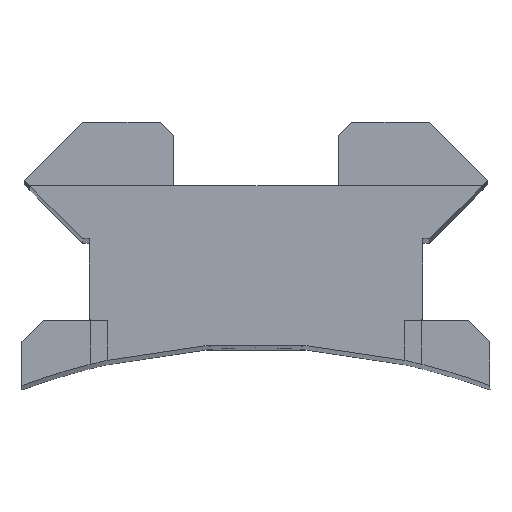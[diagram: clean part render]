
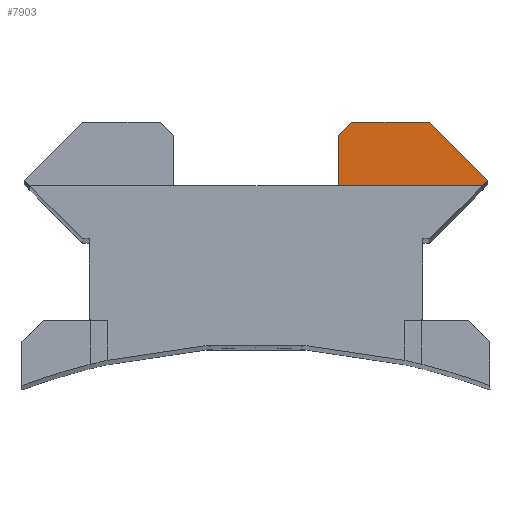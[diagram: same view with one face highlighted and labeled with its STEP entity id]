
A CAD part, top view. The second image highlights one B-rep face of the part: STEP entity #7903.
In plain terms, the highlighted planar face has unit normal (0, 0, 1).
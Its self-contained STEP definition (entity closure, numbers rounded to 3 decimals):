
#1750 = PLANE('',#1751);
#1751 = AXIS2_PLACEMENT_3D('',#1752,#1753,#1754);
#1752 = CARTESIAN_POINT('',(8.153,3.835,0.));
#1753 = DIRECTION('',(0.707,-0.707,0.));
#1754 = DIRECTION('',(0.,0.,-1.));
#2114 = PLANE('',#2115);
#2115 = AXIS2_PLACEMENT_3D('',#2116,#2117,#2118);
#2116 = CARTESIAN_POINT('',(10.897,6.325,-172.669));
#2117 = DIRECTION('',(0.,-1.,0.));
#2118 = DIRECTION('',(0.,0.,-1.));
#4170 = VERTEX_POINT('',#4171);
#4171 = CARTESIAN_POINT('',(10.897,6.579,-31.394));
#4185 = PLANE('',#4186);
#4186 = AXIS2_PLACEMENT_3D('',#4187,#4188,#4189);
#4187 = CARTESIAN_POINT('',(10.897,6.579,0.));
#4188 = DIRECTION('',(0.707,0.707,0.));
#4189 = DIRECTION('',(0.,0.,-1.));
#4197 = EDGE_CURVE('',#4170,#4198,#4200,.T.);
#4198 = VERTEX_POINT('',#4199);
#4199 = CARTESIAN_POINT('',(10.643,6.325,-31.394));
#4200 = SURFACE_CURVE('',#4201,(#4205,#4212),.PCURVE_S1.);
#4201 = LINE('',#4202,#4203);
#4202 = CARTESIAN_POINT('',(10.897,6.579,-31.394));
#4203 = VECTOR('',#4204,1.);
#4204 = DIRECTION('',(-0.707,-0.707,0.));
#4205 = PCURVE('',#1750,#4206);
#4206 = DEFINITIONAL_REPRESENTATION('',(#4207),#4211);
#4207 = LINE('',#4208,#4209);
#4208 = CARTESIAN_POINT('',(31.394,3.879));
#4209 = VECTOR('',#4210,1.);
#4210 = DIRECTION('',(0.,-1.));
#4211 = ( GEOMETRIC_REPRESENTATION_CONTEXT(2) 
PARAMETRIC_REPRESENTATION_CONTEXT() REPRESENTATION_CONTEXT('2D SPACE',''
  ) );
#4212 = PCURVE('',#4213,#4218);
#4213 = PLANE('',#4214);
#4214 = AXIS2_PLACEMENT_3D('',#4215,#4216,#4217);
#4215 = CARTESIAN_POINT('',(10.897,6.325,-31.394));
#4216 = DIRECTION('',(0.,0.,-1.));
#4217 = DIRECTION('',(-1.,0.,0.));
#4218 = DEFINITIONAL_REPRESENTATION('',(#4219),#4223);
#4219 = LINE('',#4220,#4221);
#4220 = CARTESIAN_POINT('',(0.,0.254));
#4221 = VECTOR('',#4222,1.);
#4222 = DIRECTION('',(0.707,-0.707));
#4223 = ( GEOMETRIC_REPRESENTATION_CONTEXT(2) 
PARAMETRIC_REPRESENTATION_CONTEXT() REPRESENTATION_CONTEXT('2D SPACE',''
  ) );
#5285 = VERTEX_POINT('',#5286);
#5286 = CARTESIAN_POINT('',(3.862,6.325,-31.394));
#5300 = PLANE('',#5301);
#5301 = AXIS2_PLACEMENT_3D('',#5302,#5303,#5304);
#5302 = CARTESIAN_POINT('',(3.862,6.325,0.));
#5303 = DIRECTION('',(1.,0.,0.));
#5304 = DIRECTION('',(0.,0.,-1.));
#5312 = EDGE_CURVE('',#4198,#5285,#5313,.T.);
#5313 = SURFACE_CURVE('',#5314,(#5318,#5325),.PCURVE_S1.);
#5314 = LINE('',#5315,#5316);
#5315 = CARTESIAN_POINT('',(10.643,6.325,-31.394));
#5316 = VECTOR('',#5317,1.);
#5317 = DIRECTION('',(-1.,0.,0.));
#5318 = PCURVE('',#2114,#5319);
#5319 = DEFINITIONAL_REPRESENTATION('',(#5320),#5324);
#5320 = LINE('',#5321,#5322);
#5321 = CARTESIAN_POINT('',(-141.275,-0.254));
#5322 = VECTOR('',#5323,1.);
#5323 = DIRECTION('',(0.,-1.));
#5324 = ( GEOMETRIC_REPRESENTATION_CONTEXT(2) 
PARAMETRIC_REPRESENTATION_CONTEXT() REPRESENTATION_CONTEXT('2D SPACE',''
  ) );
#5325 = PCURVE('',#4213,#5326);
#5326 = DEFINITIONAL_REPRESENTATION('',(#5327),#5331);
#5327 = LINE('',#5328,#5329);
#5328 = CARTESIAN_POINT('',(0.254,0.));
#5329 = VECTOR('',#5330,1.);
#5330 = DIRECTION('',(1.,0.));
#5331 = ( GEOMETRIC_REPRESENTATION_CONTEXT(2) 
PARAMETRIC_REPRESENTATION_CONTEXT() REPRESENTATION_CONTEXT('2D SPACE',''
  ) );
#7903 = ADVANCED_FACE('',(#7904),#4213,.F.);
#7904 = FACE_BOUND('',#7905,.T.);
#7905 = EDGE_LOOP('',(#7906,#7936,#7957,#7958,#7959,#7982));
#7906 = ORIENTED_EDGE('',*,*,#7907,.F.);
#7907 = EDGE_CURVE('',#7908,#7910,#7912,.T.);
#7908 = VERTEX_POINT('',#7909);
#7909 = CARTESIAN_POINT('',(3.862,8.687,-31.394));
#7910 = VERTEX_POINT('',#7911);
#7911 = CARTESIAN_POINT('',(4.497,9.322,-31.394));
#7912 = SURFACE_CURVE('',#7913,(#7917,#7924),.PCURVE_S1.);
#7913 = LINE('',#7914,#7915);
#7914 = CARTESIAN_POINT('',(3.862,8.687,-31.394));
#7915 = VECTOR('',#7916,1.);
#7916 = DIRECTION('',(0.707,0.707,0.));
#7917 = PCURVE('',#4213,#7918);
#7918 = DEFINITIONAL_REPRESENTATION('',(#7919),#7923);
#7919 = LINE('',#7920,#7921);
#7920 = CARTESIAN_POINT('',(7.034,2.362));
#7921 = VECTOR('',#7922,1.);
#7922 = DIRECTION('',(-0.707,0.707));
#7923 = ( GEOMETRIC_REPRESENTATION_CONTEXT(2) 
PARAMETRIC_REPRESENTATION_CONTEXT() REPRESENTATION_CONTEXT('2D SPACE',''
  ) );
#7924 = PCURVE('',#7925,#7930);
#7925 = PLANE('',#7926);
#7926 = AXIS2_PLACEMENT_3D('',#7927,#7928,#7929);
#7927 = CARTESIAN_POINT('',(4.18,9.004,0.));
#7928 = DIRECTION('',(-0.707,0.707,0.));
#7929 = DIRECTION('',(0.,0.,1.));
#7930 = DEFINITIONAL_REPRESENTATION('',(#7931),#7935);
#7931 = LINE('',#7932,#7933);
#7932 = CARTESIAN_POINT('',(-31.394,-0.449));
#7933 = VECTOR('',#7934,1.);
#7934 = DIRECTION('',(0.,1.));
#7935 = ( GEOMETRIC_REPRESENTATION_CONTEXT(2) 
PARAMETRIC_REPRESENTATION_CONTEXT() REPRESENTATION_CONTEXT('2D SPACE',''
  ) );
#7936 = ORIENTED_EDGE('',*,*,#7937,.T.);
#7937 = EDGE_CURVE('',#7908,#5285,#7938,.T.);
#7938 = SURFACE_CURVE('',#7939,(#7943,#7950),.PCURVE_S1.);
#7939 = LINE('',#7940,#7941);
#7940 = CARTESIAN_POINT('',(3.862,8.687,-31.394));
#7941 = VECTOR('',#7942,1.);
#7942 = DIRECTION('',(0.,-1.,0.));
#7943 = PCURVE('',#4213,#7944);
#7944 = DEFINITIONAL_REPRESENTATION('',(#7945),#7949);
#7945 = LINE('',#7946,#7947);
#7946 = CARTESIAN_POINT('',(7.034,2.362));
#7947 = VECTOR('',#7948,1.);
#7948 = DIRECTION('',(0.,-1.));
#7949 = ( GEOMETRIC_REPRESENTATION_CONTEXT(2) 
PARAMETRIC_REPRESENTATION_CONTEXT() REPRESENTATION_CONTEXT('2D SPACE',''
  ) );
#7950 = PCURVE('',#5300,#7951);
#7951 = DEFINITIONAL_REPRESENTATION('',(#7952),#7956);
#7952 = LINE('',#7953,#7954);
#7953 = CARTESIAN_POINT('',(31.394,2.362));
#7954 = VECTOR('',#7955,1.);
#7955 = DIRECTION('',(0.,-1.));
#7956 = ( GEOMETRIC_REPRESENTATION_CONTEXT(2) 
PARAMETRIC_REPRESENTATION_CONTEXT() REPRESENTATION_CONTEXT('2D SPACE',''
  ) );
#7957 = ORIENTED_EDGE('',*,*,#5312,.F.);
#7958 = ORIENTED_EDGE('',*,*,#4197,.F.);
#7959 = ORIENTED_EDGE('',*,*,#7960,.F.);
#7960 = EDGE_CURVE('',#7961,#4170,#7963,.T.);
#7961 = VERTEX_POINT('',#7962);
#7962 = CARTESIAN_POINT('',(8.153,9.322,-31.394));
#7963 = SURFACE_CURVE('',#7964,(#7968,#7975),.PCURVE_S1.);
#7964 = LINE('',#7965,#7966);
#7965 = CARTESIAN_POINT('',(8.153,9.322,-31.394));
#7966 = VECTOR('',#7967,1.);
#7967 = DIRECTION('',(0.707,-0.707,0.));
#7968 = PCURVE('',#4213,#7969);
#7969 = DEFINITIONAL_REPRESENTATION('',(#7970),#7974);
#7970 = LINE('',#7971,#7972);
#7971 = CARTESIAN_POINT('',(2.743,2.997));
#7972 = VECTOR('',#7973,1.);
#7973 = DIRECTION('',(-0.707,-0.707));
#7974 = ( GEOMETRIC_REPRESENTATION_CONTEXT(2) 
PARAMETRIC_REPRESENTATION_CONTEXT() REPRESENTATION_CONTEXT('2D SPACE',''
  ) );
#7975 = PCURVE('',#4185,#7976);
#7976 = DEFINITIONAL_REPRESENTATION('',(#7977),#7981);
#7977 = LINE('',#7978,#7979);
#7978 = CARTESIAN_POINT('',(31.394,3.879));
#7979 = VECTOR('',#7980,1.);
#7980 = DIRECTION('',(0.,-1.));
#7981 = ( GEOMETRIC_REPRESENTATION_CONTEXT(2) 
PARAMETRIC_REPRESENTATION_CONTEXT() REPRESENTATION_CONTEXT('2D SPACE',''
  ) );
#7982 = ORIENTED_EDGE('',*,*,#7983,.F.);
#7983 = EDGE_CURVE('',#7910,#7961,#7984,.T.);
#7984 = SURFACE_CURVE('',#7985,(#7989,#7996),.PCURVE_S1.);
#7985 = LINE('',#7986,#7987);
#7986 = CARTESIAN_POINT('',(4.497,9.322,-31.394));
#7987 = VECTOR('',#7988,1.);
#7988 = DIRECTION('',(1.,0.,0.));
#7989 = PCURVE('',#4213,#7990);
#7990 = DEFINITIONAL_REPRESENTATION('',(#7991),#7995);
#7991 = LINE('',#7992,#7993);
#7992 = CARTESIAN_POINT('',(6.399,2.997));
#7993 = VECTOR('',#7994,1.);
#7994 = DIRECTION('',(-1.,0.));
#7995 = ( GEOMETRIC_REPRESENTATION_CONTEXT(2) 
PARAMETRIC_REPRESENTATION_CONTEXT() REPRESENTATION_CONTEXT('2D SPACE',''
  ) );
#7996 = PCURVE('',#7997,#8002);
#7997 = PLANE('',#7998);
#7998 = AXIS2_PLACEMENT_3D('',#7999,#8000,#8001);
#7999 = CARTESIAN_POINT('',(8.153,9.322,0.));
#8000 = DIRECTION('',(0.,1.,0.));
#8001 = DIRECTION('',(0.,0.,1.));
#8002 = DEFINITIONAL_REPRESENTATION('',(#8003),#8007);
#8003 = LINE('',#8004,#8005);
#8004 = CARTESIAN_POINT('',(-31.394,-3.656));
#8005 = VECTOR('',#8006,1.);
#8006 = DIRECTION('',(0.,1.));
#8007 = ( GEOMETRIC_REPRESENTATION_CONTEXT(2) 
PARAMETRIC_REPRESENTATION_CONTEXT() REPRESENTATION_CONTEXT('2D SPACE',''
  ) );
